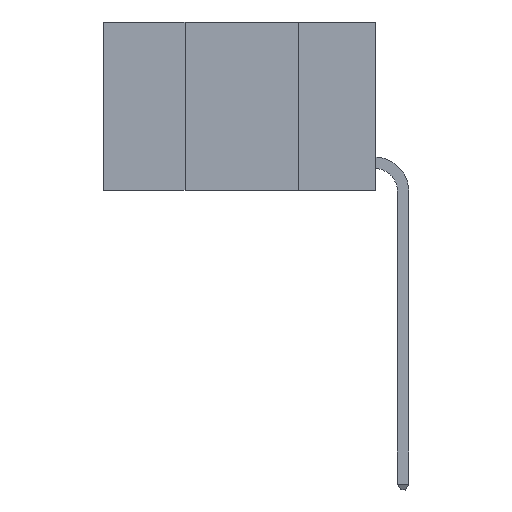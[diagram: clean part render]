
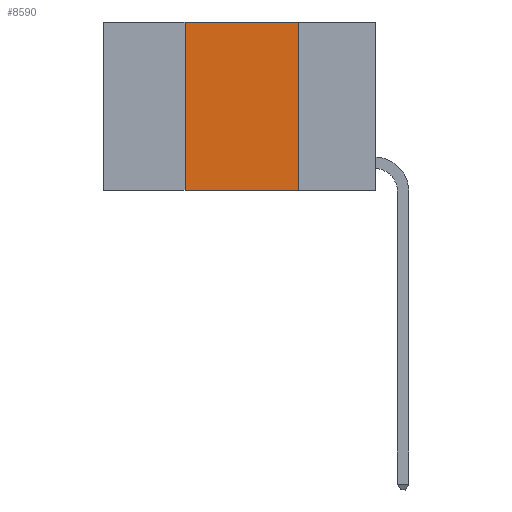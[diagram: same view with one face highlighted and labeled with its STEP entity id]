
A CAD part, left-side view. The second image highlights one B-rep face of the part: STEP entity #8590.
In plain terms, the highlighted planar face has unit normal (-1, 0, 0).
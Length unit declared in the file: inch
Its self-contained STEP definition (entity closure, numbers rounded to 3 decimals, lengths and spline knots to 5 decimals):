
#614 = EDGE_CURVE ( 'NONE', #1656, #9046, #10678, .T. ) ;
#931 = DIRECTION ( 'NONE',  ( 0., 0., 1. ) ) ;
#1055 = VERTEX_POINT ( 'NONE', #6761 ) ;
#1465 = LINE ( 'NONE', #8603, #3507 ) ;
#1574 = LINE ( 'NONE', #5159, #6172 ) ;
#1656 = VERTEX_POINT ( 'NONE', #3712 ) ;
#1846 = VECTOR ( 'NONE', #5191, 39.37008 ) ;
#2115 = FACE_OUTER_BOUND ( 'NONE', #2596, .T. ) ;
#2155 = CARTESIAN_POINT ( 'NONE',  ( 0., 0.6, 0. ) ) ;
#2593 = CARTESIAN_POINT ( 'NONE',  ( 0., 0.6, -0.37 ) ) ;
#2596 = EDGE_LOOP ( 'NONE', ( #5014, #5225, #5226, #5288 ) ) ;
#2721 = VERTEX_POINT ( 'NONE', #9272 ) ;
#3349 = EDGE_CURVE ( 'NONE', #2721, #9046, #6960, .T. ) ;
#3507 = VECTOR ( 'NONE', #931, 39.37008 ) ;
#3712 = CARTESIAN_POINT ( 'NONE',  ( 0., 0.42, -0.37 ) ) ;
#4784 = DIRECTION ( 'NONE',  ( 1., 0., 0. ) ) ;
#5014 = ORIENTED_EDGE ( 'NONE', *, *, #3349, .F. ) ;
#5159 = CARTESIAN_POINT ( 'NONE',  ( 0., 0.6, 0. ) ) ;
#5191 = DIRECTION ( 'NONE',  ( 0., 0., -1. ) ) ;
#5225 = ORIENTED_EDGE ( 'NONE', *, *, #8228, .F. ) ;
#5226 = ORIENTED_EDGE ( 'NONE', *, *, #7153, .F. ) ;
#5288 = ORIENTED_EDGE ( 'NONE', *, *, #614, .T. ) ;
#5563 = DIRECTION ( 'NONE',  ( 0., -1., 0. ) ) ;
#6019 = CARTESIAN_POINT ( 'NONE',  ( 0., 0.17, 0. ) ) ;
#6172 = VECTOR ( 'NONE', #6851, 39.37008 ) ;
#6761 = CARTESIAN_POINT ( 'NONE',  ( 0., 0.42, 0. ) ) ;
#6851 = DIRECTION ( 'NONE',  ( 0., -1., 0. ) ) ;
#6960 = LINE ( 'NONE', #6019, #1846 ) ;
#7153 = EDGE_CURVE ( 'NONE', #1656, #1055, #1465, .T. ) ;
#8228 = EDGE_CURVE ( 'NONE', #1055, #2721, #1574, .T. ) ;
#8544 = VECTOR ( 'NONE', #5563, 39.37008 ) ;
#8590 = ADVANCED_FACE ( 'NONE', ( #2115 ), #9731, .F. ) ;
#8603 = CARTESIAN_POINT ( 'NONE',  ( 0., 0.42, 0. ) ) ;
#9046 = VERTEX_POINT ( 'NONE', #9505 ) ;
#9272 = CARTESIAN_POINT ( 'NONE',  ( 0., 0.17, 0. ) ) ;
#9505 = CARTESIAN_POINT ( 'NONE',  ( 0., 0.17, -0.37 ) ) ;
#9731 = PLANE ( 'NONE',  #10898 ) ;
#10545 = DIRECTION ( 'NONE',  ( 0., 0., -1. ) ) ;
#10678 = LINE ( 'NONE', #2593, #8544 ) ;
#10898 = AXIS2_PLACEMENT_3D ( 'NONE', #2155, #4784, #10545 ) ;
